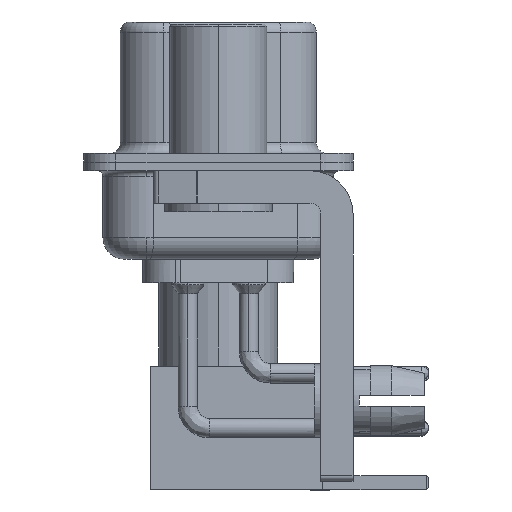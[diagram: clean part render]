
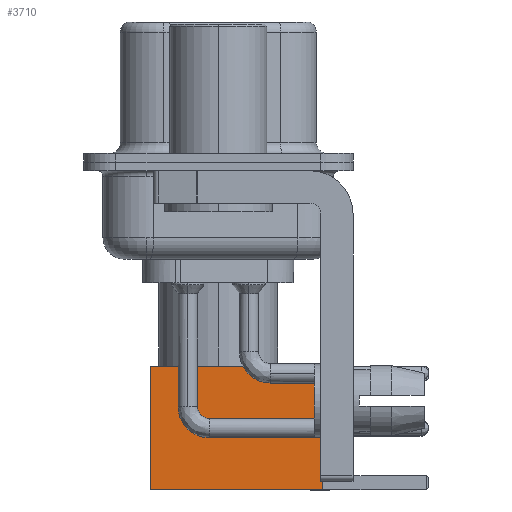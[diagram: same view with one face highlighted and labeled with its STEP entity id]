
A CAD part, left-side view. The second image highlights one B-rep face of the part: STEP entity #3710.
In plain terms, the highlighted face is planar.
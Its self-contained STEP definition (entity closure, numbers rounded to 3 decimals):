
#894 = ORIENTED_EDGE ( 'NONE', *, *, #12939, .F. ) ;
#1153 = LINE ( 'NONE', #13540, #15957 ) ;
#1464 = VERTEX_POINT ( 'NONE', #17497 ) ;
#1525 = EDGE_CURVE ( 'NONE', #1464, #9855, #7831, .T. ) ;
#3710 = ADVANCED_FACE ( 'NONE', ( #25697 ), #13241, .T. ) ;
#4030 = DIRECTION ( 'NONE',  ( 0., 0., -1. ) ) ;
#4443 = AXIS2_PLACEMENT_3D ( 'NONE', #9137, #22044, #23545 ) ;
#4996 = DIRECTION ( 'NONE',  ( -1., 0., 0. ) ) ;
#6928 = VECTOR ( 'NONE', #24936, 1000. ) ;
#7350 = VECTOR ( 'NONE', #4030, 1000. ) ;
#7831 = LINE ( 'NONE', #14098, #7350 ) ;
#8017 = VERTEX_POINT ( 'NONE', #24340 ) ;
#8506 = CARTESIAN_POINT ( 'NONE',  ( -2.875, 2.875, 0. ) ) ;
#9137 = CARTESIAN_POINT ( 'NONE',  ( 2.875, 2.875, 0. ) ) ;
#9704 = EDGE_LOOP ( 'NONE', ( #23679, #26018, #14219, #894 ) ) ;
#9855 = VERTEX_POINT ( 'NONE', #8506 ) ;
#11321 = EDGE_CURVE ( 'NONE', #8017, #18574, #1153, .T. ) ;
#11643 = LINE ( 'NONE', #19934, #25154 ) ;
#11891 = DIRECTION ( 'NONE',  ( 0., 0., -1. ) ) ;
#12939 = EDGE_CURVE ( 'NONE', #8017, #1464, #17079, .T. ) ;
#13241 = PLANE ( 'NONE',  #4443 ) ;
#13540 = CARTESIAN_POINT ( 'NONE',  ( 2.875, 2.875, 0. ) ) ;
#14098 = CARTESIAN_POINT ( 'NONE',  ( -2.875, 2.875, 0. ) ) ;
#14219 = ORIENTED_EDGE ( 'NONE', *, *, #1525, .F. ) ;
#15021 = EDGE_CURVE ( 'NONE', #18574, #9855, #11643, .T. ) ;
#15957 = VECTOR ( 'NONE', #11891, 1000. ) ;
#17079 = LINE ( 'NONE', #25205, #6928 ) ;
#17497 = CARTESIAN_POINT ( 'NONE',  ( -2.875, 2.875, 8. ) ) ;
#18574 = VERTEX_POINT ( 'NONE', #18844 ) ;
#18844 = CARTESIAN_POINT ( 'NONE',  ( 2.875, 2.875, 0. ) ) ;
#19934 = CARTESIAN_POINT ( 'NONE',  ( 0., 2.875, 0. ) ) ;
#22044 = DIRECTION ( 'NONE',  ( 0., 1., 0. ) ) ;
#23545 = DIRECTION ( 'NONE',  ( 0., 0., 1. ) ) ;
#23679 = ORIENTED_EDGE ( 'NONE', *, *, #11321, .T. ) ;
#24340 = CARTESIAN_POINT ( 'NONE',  ( 2.875, 2.875, 8. ) ) ;
#24936 = DIRECTION ( 'NONE',  ( -1., 0., 0. ) ) ;
#25154 = VECTOR ( 'NONE', #4996, 1000. ) ;
#25205 = CARTESIAN_POINT ( 'NONE',  ( 0., 2.875, 8. ) ) ;
#25697 = FACE_OUTER_BOUND ( 'NONE', #9704, .T. ) ;
#26018 = ORIENTED_EDGE ( 'NONE', *, *, #15021, .T. ) ;
